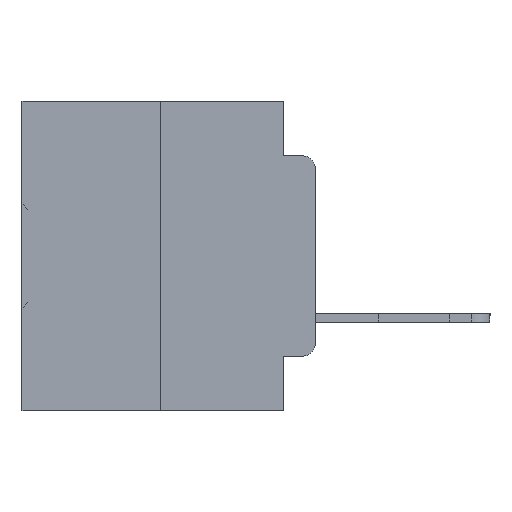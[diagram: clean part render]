
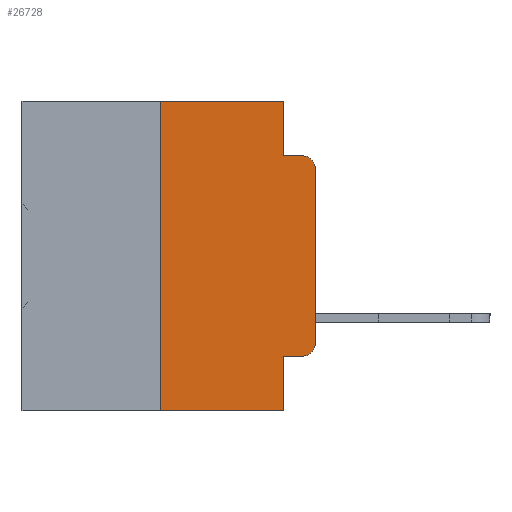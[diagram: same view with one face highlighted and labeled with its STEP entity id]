
A CAD part, left-side view. The second image highlights one B-rep face of the part: STEP entity #26728.
In plain terms, the highlighted planar face has unit normal (-1, 0, 0).
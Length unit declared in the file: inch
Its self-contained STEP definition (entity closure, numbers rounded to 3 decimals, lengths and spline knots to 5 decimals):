
#266 = CARTESIAN_POINT ( 'NONE',  ( 0., 0.02, -0.3915 ) ) ;
#422 = CARTESIAN_POINT ( 'NONE',  ( 0., 0.051, -0.5 ) ) ;
#1052 = VERTEX_POINT ( 'NONE', #2188 ) ;
#1846 = VERTEX_POINT ( 'NONE', #422 ) ;
#1936 = CARTESIAN_POINT ( 'NONE',  ( 0., 0.02, -0.1085 ) ) ;
#2188 = CARTESIAN_POINT ( 'NONE',  ( 0., 0.25, 0. ) ) ;
#2258 = EDGE_CURVE ( 'NONE', #28835, #1052, #15435, .T. ) ;
#2852 = VERTEX_POINT ( 'NONE', #33471 ) ;
#3101 = DIRECTION ( 'NONE',  ( 0., 0., -1. ) ) ;
#4003 = LINE ( 'NONE', #24106, #34798 ) ;
#4009 = CARTESIAN_POINT ( 'NONE',  ( 0., 0.051, -0.0885 ) ) ;
#4477 = EDGE_CURVE ( 'NONE', #2852, #13566, #4003, .T. ) ;
#4532 = LINE ( 'NONE', #4009, #18670 ) ;
#4824 = DIRECTION ( 'NONE',  ( 0., 0., -1. ) ) ;
#5111 = DIRECTION ( 'NONE',  ( 0., 0., 1. ) ) ;
#5587 = PLANE ( 'NONE',  #17902 ) ;
#6021 = CARTESIAN_POINT ( 'NONE',  ( 0., 0.25, -0.5 ) ) ;
#6431 = EDGE_CURVE ( 'NONE', #13566, #28441, #12711, .T. ) ;
#6700 = LINE ( 'NONE', #12243, #28241 ) ;
#6813 = VECTOR ( 'NONE', #33494, 39.37008 ) ;
#7268 = DIRECTION ( 'NONE',  ( 0., 0., 1. ) ) ;
#7553 = LINE ( 'NONE', #13489, #22525 ) ;
#8084 = EDGE_CURVE ( 'NONE', #32298, #34243, #9466, .T. ) ;
#8438 = DIRECTION ( 'NONE',  ( 1., 0., 0. ) ) ;
#9347 = DIRECTION ( 'NONE',  ( 0., 0., -1. ) ) ;
#9466 = LINE ( 'NONE', #27837, #6813 ) ;
#9746 = CARTESIAN_POINT ( 'NONE',  ( 0., 0.02, -0.0885 ) ) ;
#10582 = ORIENTED_EDGE ( 'NONE', *, *, #17618, .T. ) ;
#10816 = EDGE_CURVE ( 'NONE', #28835, #1846, #7553, .T. ) ;
#11309 = AXIS2_PLACEMENT_3D ( 'NONE', #1936, #21683, #4824 ) ;
#11800 = EDGE_CURVE ( 'NONE', #32298, #1846, #33853, .T. ) ;
#12243 = CARTESIAN_POINT ( 'NONE',  ( 0., 0.051, 0. ) ) ;
#12711 = CIRCLE ( 'NONE', #11309, 0.02 ) ;
#13489 = CARTESIAN_POINT ( 'NONE',  ( 0., 0.473, -0.5 ) ) ;
#13566 = VERTEX_POINT ( 'NONE', #36267 ) ;
#14702 = ORIENTED_EDGE ( 'NONE', *, *, #4477, .T. ) ;
#15435 = LINE ( 'NONE', #30442, #29456 ) ;
#15625 = ORIENTED_EDGE ( 'NONE', *, *, #21821, .F. ) ;
#15691 = FACE_OUTER_BOUND ( 'NONE', #32868, .T. ) ;
#17618 = EDGE_CURVE ( 'NONE', #34243, #2852, #30365, .T. ) ;
#17773 = CARTESIAN_POINT ( 'NONE',  ( 0., 0.051, 0. ) ) ;
#17902 = AXIS2_PLACEMENT_3D ( 'NONE', #25245, #8438, #28069 ) ;
#18063 = ORIENTED_EDGE ( 'NONE', *, *, #36173, .F. ) ;
#18614 = CARTESIAN_POINT ( 'NONE',  ( 0., 0.473, 0. ) ) ;
#18670 = VECTOR ( 'NONE', #23697, 39.37008 ) ;
#18729 = DIRECTION ( 'NONE',  ( 0., -1., 0. ) ) ;
#20015 = DIRECTION ( 'NONE',  ( -1., 0., 0. ) ) ;
#20973 = CARTESIAN_POINT ( 'NONE',  ( 0., 0.02, -0.4115 ) ) ;
#21275 = EDGE_CURVE ( 'NONE', #29919, #28441, #4532, .T. ) ;
#21683 = DIRECTION ( 'NONE',  ( -1., 0., 0. ) ) ;
#21700 = LINE ( 'NONE', #18614, #35719 ) ;
#21821 = EDGE_CURVE ( 'NONE', #22622, #29919, #6700, .T. ) ;
#22525 = VECTOR ( 'NONE', #33148, 39.37008 ) ;
#22622 = VERTEX_POINT ( 'NONE', #31904 ) ;
#22883 = AXIS2_PLACEMENT_3D ( 'NONE', #266, #20015, #3101 ) ;
#23697 = DIRECTION ( 'NONE',  ( 0., -1., 0. ) ) ;
#24106 = CARTESIAN_POINT ( 'NONE',  ( 0., 0., 0. ) ) ;
#25245 = CARTESIAN_POINT ( 'NONE',  ( 0., 0.473, 0. ) ) ;
#25473 = CARTESIAN_POINT ( 'NONE',  ( 0., 0.051, -0.0885 ) ) ;
#26197 = ORIENTED_EDGE ( 'NONE', *, *, #8084, .T. ) ;
#26384 = VECTOR ( 'NONE', #9347, 39.37008 ) ;
#26728 = ADVANCED_FACE ( 'NONE', ( #15691 ), #5587, .F. ) ;
#27837 = CARTESIAN_POINT ( 'NONE',  ( 0., 0.051, -0.4115 ) ) ;
#28069 = DIRECTION ( 'NONE',  ( 0., 0., -1. ) ) ;
#28241 = VECTOR ( 'NONE', #34694, 39.37008 ) ;
#28441 = VERTEX_POINT ( 'NONE', #9746 ) ;
#28835 = VERTEX_POINT ( 'NONE', #6021 ) ;
#29456 = VECTOR ( 'NONE', #5111, 39.37008 ) ;
#29478 = ORIENTED_EDGE ( 'NONE', *, *, #21275, .F. ) ;
#29919 = VERTEX_POINT ( 'NONE', #25473 ) ;
#30365 = CIRCLE ( 'NONE', #22883, 0.02 ) ;
#30442 = CARTESIAN_POINT ( 'NONE',  ( 0., 0.25, 0. ) ) ;
#30506 = CARTESIAN_POINT ( 'NONE',  ( 0., 0.051, -0.4115 ) ) ;
#30813 = ORIENTED_EDGE ( 'NONE', *, *, #11800, .F. ) ;
#31904 = CARTESIAN_POINT ( 'NONE',  ( 0., 0.051, 0. ) ) ;
#32298 = VERTEX_POINT ( 'NONE', #30506 ) ;
#32868 = EDGE_LOOP ( 'NONE', ( #14702, #34894, #29478, #15625, #18063, #35092, #33477, #30813, #26197, #10582 ) ) ;
#33148 = DIRECTION ( 'NONE',  ( 0., -1., 0. ) ) ;
#33471 = CARTESIAN_POINT ( 'NONE',  ( 0., 0., -0.3915 ) ) ;
#33477 = ORIENTED_EDGE ( 'NONE', *, *, #10816, .T. ) ;
#33494 = DIRECTION ( 'NONE',  ( 0., -1., 0. ) ) ;
#33853 = LINE ( 'NONE', #17773, #26384 ) ;
#34243 = VERTEX_POINT ( 'NONE', #20973 ) ;
#34694 = DIRECTION ( 'NONE',  ( 0., 0., -1. ) ) ;
#34798 = VECTOR ( 'NONE', #7268, 39.37008 ) ;
#34894 = ORIENTED_EDGE ( 'NONE', *, *, #6431, .T. ) ;
#35092 = ORIENTED_EDGE ( 'NONE', *, *, #2258, .F. ) ;
#35719 = VECTOR ( 'NONE', #18729, 39.37008 ) ;
#36173 = EDGE_CURVE ( 'NONE', #1052, #22622, #21700, .T. ) ;
#36267 = CARTESIAN_POINT ( 'NONE',  ( 0., 0., -0.1085 ) ) ;
